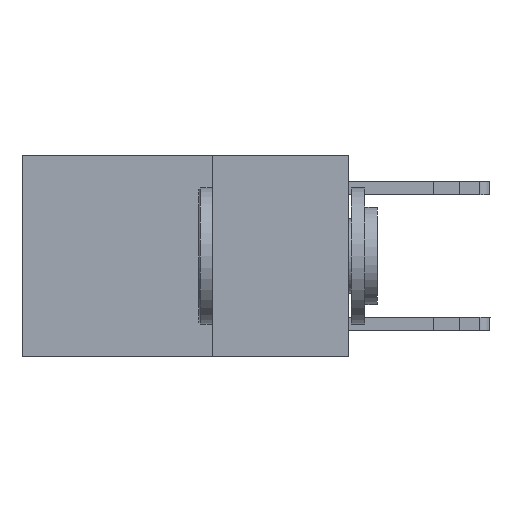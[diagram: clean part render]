
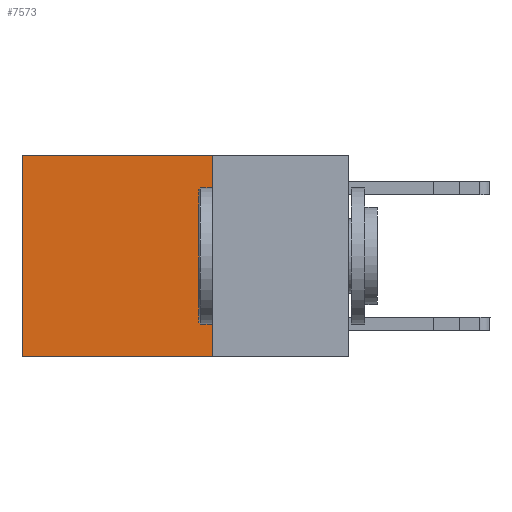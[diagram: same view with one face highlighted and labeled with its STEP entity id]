
A CAD part, left-side view. The second image highlights one B-rep face of the part: STEP entity #7573.
In plain terms, the highlighted planar face has unit normal (-1, 0, 0).
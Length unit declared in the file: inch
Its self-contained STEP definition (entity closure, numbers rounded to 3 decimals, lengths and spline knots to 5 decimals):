
#7 = CARTESIAN_POINT ( 'NONE',  ( 0.2625, 0.25, 0. ) ) ;
#537 = DIRECTION ( 'NONE',  ( 0., 1., 0. ) ) ;
#966 = VECTOR ( 'NONE', #14134, 39.37008 ) ;
#1327 = LINE ( 'NONE', #2044, #966 ) ;
#1587 = CARTESIAN_POINT ( 'NONE',  ( 0.2625, 0.6, -0.37 ) ) ;
#1918 = EDGE_CURVE ( 'NONE', #16367, #9957, #1327, .T. ) ;
#2044 = CARTESIAN_POINT ( 'NONE',  ( 0.2625, 0.25, -0.37 ) ) ;
#2207 = CARTESIAN_POINT ( 'NONE',  ( 0.2625, 0.25, 0. ) ) ;
#3447 = DIRECTION ( 'NONE',  ( 0., 0., -1. ) ) ;
#3451 = CARTESIAN_POINT ( 'NONE',  ( 0.2625, 0.6, 0. ) ) ;
#3461 = CARTESIAN_POINT ( 'NONE',  ( 0.2625, 0.25, -0.37 ) ) ;
#4176 = FACE_OUTER_BOUND ( 'NONE', #13867, .T. ) ;
#4359 = EDGE_CURVE ( 'NONE', #12706, #16367, #9133, .T. ) ;
#5173 = LINE ( 'NONE', #7, #5416 ) ;
#5416 = VECTOR ( 'NONE', #537, 39.37008 ) ;
#5656 = CARTESIAN_POINT ( 'NONE',  ( 0.2625, 0.6, 0. ) ) ;
#6376 = EDGE_CURVE ( 'NONE', #18922, #9957, #18915, .T. ) ;
#7344 = DIRECTION ( 'NONE',  ( 0., 0., -1. ) ) ;
#7347 = DIRECTION ( 'NONE',  ( 1., 0., 0. ) ) ;
#7573 = ADVANCED_FACE ( 'NONE', ( #4176 ), #8165, .F. ) ;
#7867 = ORIENTED_EDGE ( 'NONE', *, *, #1918, .F. ) ;
#8165 = PLANE ( 'NONE',  #13432 ) ;
#8259 = CARTESIAN_POINT ( 'NONE',  ( 0.2625, 0.25, 0. ) ) ;
#9002 = VECTOR ( 'NONE', #11341, 39.37008 ) ;
#9133 = LINE ( 'NONE', #11256, #9002 ) ;
#9957 = VERTEX_POINT ( 'NONE', #1587 ) ;
#10801 = ORIENTED_EDGE ( 'NONE', *, *, #4359, .F. ) ;
#11256 = CARTESIAN_POINT ( 'NONE',  ( 0.2625, 0.25, 0. ) ) ;
#11341 = DIRECTION ( 'NONE',  ( 0., 0., -1. ) ) ;
#11653 = ORIENTED_EDGE ( 'NONE', *, *, #15248, .T. ) ;
#12706 = VERTEX_POINT ( 'NONE', #2207 ) ;
#13432 = AXIS2_PLACEMENT_3D ( 'NONE', #8259, #7347, #7344 ) ;
#13867 = EDGE_LOOP ( 'NONE', ( #17732, #7867, #10801, #11653 ) ) ;
#14134 = DIRECTION ( 'NONE',  ( 0., 1., 0. ) ) ;
#15248 = EDGE_CURVE ( 'NONE', #12706, #18922, #5173, .T. ) ;
#16367 = VERTEX_POINT ( 'NONE', #3461 ) ;
#17732 = ORIENTED_EDGE ( 'NONE', *, *, #6376, .T. ) ;
#18915 = LINE ( 'NONE', #3451, #19580 ) ;
#18922 = VERTEX_POINT ( 'NONE', #5656 ) ;
#19580 = VECTOR ( 'NONE', #3447, 39.37008 ) ;
